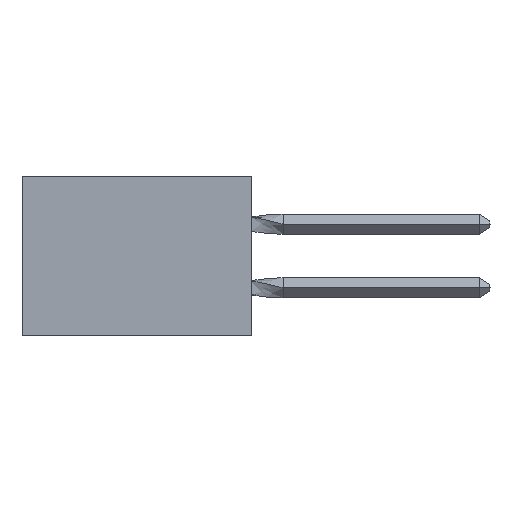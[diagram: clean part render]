
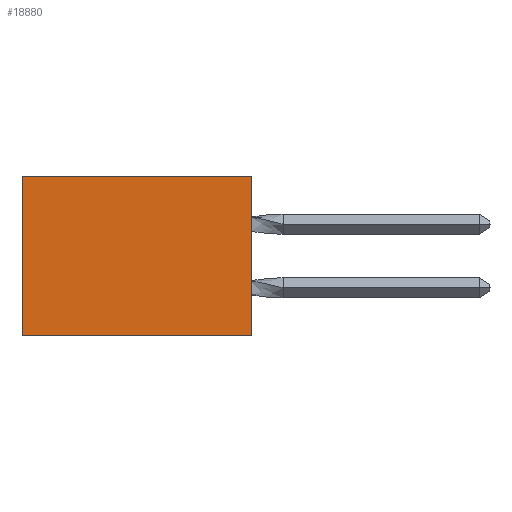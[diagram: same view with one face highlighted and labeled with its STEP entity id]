
A CAD part, left-side view. The second image highlights one B-rep face of the part: STEP entity #18880.
In plain terms, the highlighted planar face has unit normal (-1, 0, 0).
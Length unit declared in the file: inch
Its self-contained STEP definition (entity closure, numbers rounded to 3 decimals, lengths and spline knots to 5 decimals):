
#1089 = ORIENTED_EDGE ( 'NONE', *, *, #26040, .T. ) ;
#2708 = EDGE_CURVE ( 'NONE', #6632, #11233, #29195, .T. ) ;
#5818 = DIRECTION ( 'NONE',  ( 0., 0., -1. ) ) ;
#5878 = DIRECTION ( 'NONE',  ( 0., 1., 0. ) ) ;
#5996 = EDGE_CURVE ( 'NONE', #7236, #20513, #28245, .T. ) ;
#6096 = LINE ( 'NONE', #18396, #7214 ) ;
#6632 = VERTEX_POINT ( 'NONE', #30369 ) ;
#7095 = FACE_OUTER_BOUND ( 'NONE', #24855, .T. ) ;
#7214 = VECTOR ( 'NONE', #25467, 39.37008 ) ;
#7236 = VERTEX_POINT ( 'NONE', #24151 ) ;
#7804 = ORIENTED_EDGE ( 'NONE', *, *, #5996, .T. ) ;
#8357 = CARTESIAN_POINT ( 'NONE',  ( 0.305, 0., -0.5 ) ) ;
#8793 = CARTESIAN_POINT ( 'NONE',  ( 0.305, 0., -0.5 ) ) ;
#10405 = VECTOR ( 'NONE', #12194, 39.37008 ) ;
#11233 = VERTEX_POINT ( 'NONE', #8793 ) ;
#12194 = DIRECTION ( 'NONE',  ( 0., 0., -1. ) ) ;
#12841 = CARTESIAN_POINT ( 'NONE',  ( 0.305, 0., 0. ) ) ;
#13086 = DIRECTION ( 'NONE',  ( 1., 0., 0. ) ) ;
#14627 = DIRECTION ( 'NONE',  ( 0., 0., -1. ) ) ;
#15884 = ORIENTED_EDGE ( 'NONE', *, *, #2708, .F. ) ;
#17079 = LINE ( 'NONE', #12841, #27325 ) ;
#17524 = PLANE ( 'NONE',  #20152 ) ;
#18396 = CARTESIAN_POINT ( 'NONE',  ( 0.305, 0., -0.5 ) ) ;
#18880 = ADVANCED_FACE ( 'NONE', ( #7095 ), #17524, .F. ) ;
#20152 = AXIS2_PLACEMENT_3D ( 'NONE', #8357, #13086, #5818 ) ;
#20513 = VERTEX_POINT ( 'NONE', #27074 ) ;
#24151 = CARTESIAN_POINT ( 'NONE',  ( 0.305, 0.72, 0. ) ) ;
#24489 = EDGE_CURVE ( 'NONE', #11233, #20513, #6096, .T. ) ;
#24855 = EDGE_LOOP ( 'NONE', ( #7804, #26930, #15884, #1089 ) ) ;
#25467 = DIRECTION ( 'NONE',  ( 0., 1., 0. ) ) ;
#25872 = CARTESIAN_POINT ( 'NONE',  ( 0.305, 0., -0.5 ) ) ;
#26040 = EDGE_CURVE ( 'NONE', #6632, #7236, #17079, .T. ) ;
#26325 = CARTESIAN_POINT ( 'NONE',  ( 0.305, 0.72, -0.5 ) ) ;
#26930 = ORIENTED_EDGE ( 'NONE', *, *, #24489, .F. ) ;
#27074 = CARTESIAN_POINT ( 'NONE',  ( 0.305, 0.72, -0.5 ) ) ;
#27325 = VECTOR ( 'NONE', #5878, 39.37008 ) ;
#28245 = LINE ( 'NONE', #26325, #29362 ) ;
#29195 = LINE ( 'NONE', #25872, #10405 ) ;
#29362 = VECTOR ( 'NONE', #14627, 39.37008 ) ;
#30369 = CARTESIAN_POINT ( 'NONE',  ( 0.305, 0., 0. ) ) ;
